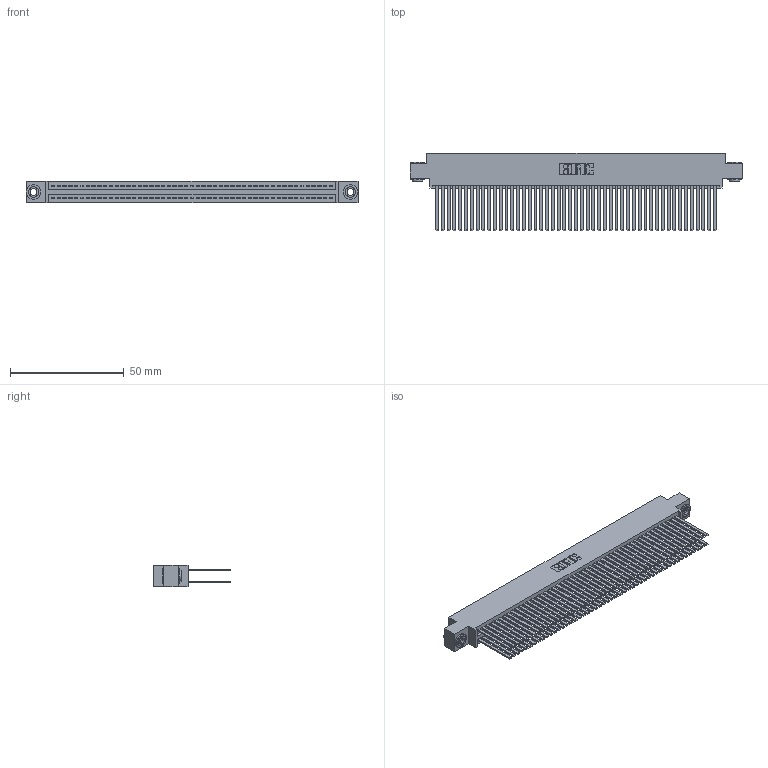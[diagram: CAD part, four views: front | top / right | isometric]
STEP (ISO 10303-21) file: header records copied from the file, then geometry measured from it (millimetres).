
FILE_DESCRIPTION (( 'STEP AP203' ), '1' );
FILE_NAME ('345-098-544-803.STEP', '2018-10-05T10:37:54', ( '' ), ( '' ), 'SwSTEP 2.0', 'SolidWorks 2016', '' );
FILE_SCHEMA (( 'CONFIG_CONTROL_DESIGN' ));
Length unit declared in the file: inch
Products named in the file (4): 345-098-544-803; 345 Part_0.170 Offset - 0.156 Dia-TH; 345-292-001_345-293-144; 345-250-002_345-250-002-102
Assembly tree (101 placements, depth 2):
  345-098-544-803
    345 Part_0.170 Offset - 0.156 Dia-TH
    345-292-001_345-293-144  x98
    345-250-002_345-250-002-102  x2
Bounding box: 145.67 x 33.96 x 9.4 mm (x, y, z)
Volume: 15495.2 mm3; surface area: 27414.9 mm2
Topology: 101 solids, 101 shells, 4480 faces, 13267 edges, 8710 vertices
Faces by surface type: plane 2936, cylinder 1536, cone 8
Entity records: 38102 total; most frequent: CARTESIAN_POINT 6355, ORIENTED_EDGE 6282, DIRECTION 5623, EDGE_CURVE 3141, VECTOR 2793, LINE 2793, VERTEX_POINT 2090, AXIS2_PLACEMENT_3D 1415
